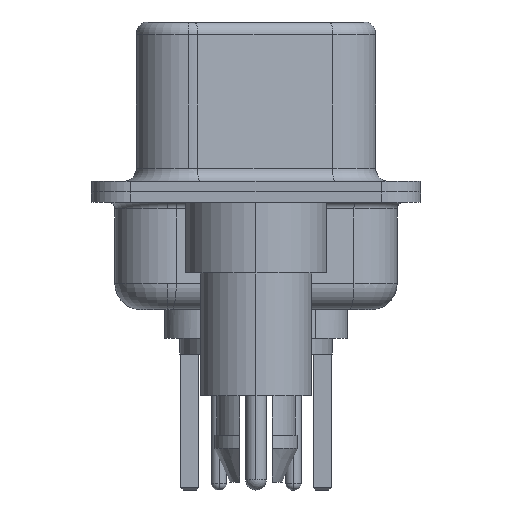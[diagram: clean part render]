
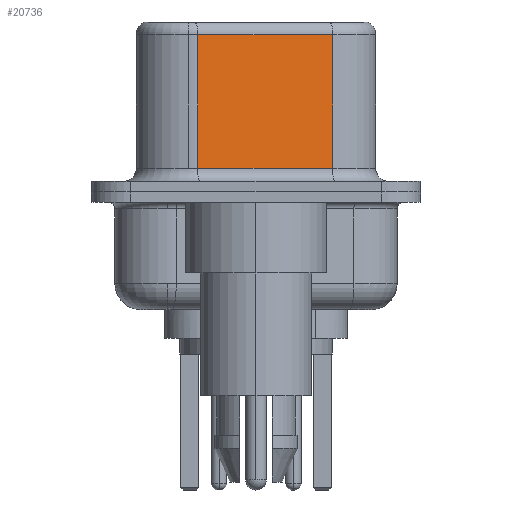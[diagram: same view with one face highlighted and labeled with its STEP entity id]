
A CAD part, left-side view. The second image highlights one B-rep face of the part: STEP entity #20736.
In plain terms, the highlighted planar face has unit normal (-0.985, -0.174, 0).
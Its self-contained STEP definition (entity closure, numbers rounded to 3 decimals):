
#952 = LINE ( 'NONE', #5443, #6398 ) ;
#957 = VERTEX_POINT ( 'NONE', #14976 ) ;
#1840 = ORIENTED_EDGE ( 'NONE', *, *, #23921, .F. ) ;
#2312 = LINE ( 'NONE', #18005, #7089 ) ;
#3660 = CARTESIAN_POINT ( 'NONE',  ( 4.585, -2.927, 6.52 ) ) ;
#3923 = VECTOR ( 'NONE', #5206, 1000. ) ;
#5206 = DIRECTION ( 'NONE',  ( 0.174, -0.985, 0. ) ) ;
#5425 = CARTESIAN_POINT ( 'NONE',  ( 3.675, 2.233, 0.9 ) ) ;
#5443 = CARTESIAN_POINT ( 'NONE',  ( 4.585, -2.927, 6.02 ) ) ;
#6398 = VECTOR ( 'NONE', #19415, 1000. ) ;
#6472 = ORIENTED_EDGE ( 'NONE', *, *, #9262, .T. ) ;
#7089 = VECTOR ( 'NONE', #19938, 1000. ) ;
#7712 = DIRECTION ( 'NONE',  ( 0.985, 0.174, 0. ) ) ;
#9262 = EDGE_CURVE ( 'NONE', #25026, #15234, #14582, .T. ) ;
#9310 = EDGE_LOOP ( 'NONE', ( #1840, #21559, #18121, #6472 ) ) ;
#11411 = EDGE_CURVE ( 'NONE', #957, #14250, #952, .T. ) ;
#12426 = LINE ( 'NONE', #25499, #17782 ) ;
#14250 = VERTEX_POINT ( 'NONE', #24524 ) ;
#14582 = LINE ( 'NONE', #15014, #3923 ) ;
#14976 = CARTESIAN_POINT ( 'NONE',  ( 4.585, -2.927, 6.02 ) ) ;
#15014 = CARTESIAN_POINT ( 'NONE',  ( 4.585, -2.927, 0.9 ) ) ;
#15234 = VERTEX_POINT ( 'NONE', #23874 ) ;
#15509 = DIRECTION ( 'NONE',  ( 0., 0., -1. ) ) ;
#17782 = VECTOR ( 'NONE', #15509, 1000. ) ;
#18005 = CARTESIAN_POINT ( 'NONE',  ( 4.585, -2.927, 6.52 ) ) ;
#18121 = ORIENTED_EDGE ( 'NONE', *, *, #22821, .T. ) ;
#18770 = FACE_OUTER_BOUND ( 'NONE', #9310, .T. ) ;
#19415 = DIRECTION ( 'NONE',  ( -0.174, 0.985, 0. ) ) ;
#19938 = DIRECTION ( 'NONE',  ( 0., 0., -1. ) ) ;
#20736 = ADVANCED_FACE ( 'NONE', ( #18770 ), #21516, .F. ) ;
#21516 = PLANE ( 'NONE',  #25714 ) ;
#21559 = ORIENTED_EDGE ( 'NONE', *, *, #11411, .T. ) ;
#21603 = DIRECTION ( 'NONE',  ( -0.174, 0.985, 0. ) ) ;
#22821 = EDGE_CURVE ( 'NONE', #14250, #25026, #12426, .T. ) ;
#23874 = CARTESIAN_POINT ( 'NONE',  ( 4.585, -2.927, 0.9 ) ) ;
#23921 = EDGE_CURVE ( 'NONE', #957, #15234, #2312, .T. ) ;
#24524 = CARTESIAN_POINT ( 'NONE',  ( 3.675, 2.233, 6.02 ) ) ;
#25026 = VERTEX_POINT ( 'NONE', #5425 ) ;
#25499 = CARTESIAN_POINT ( 'NONE',  ( 3.675, 2.233, 6.52 ) ) ;
#25714 = AXIS2_PLACEMENT_3D ( 'NONE', #3660, #7712, #21603 ) ;
